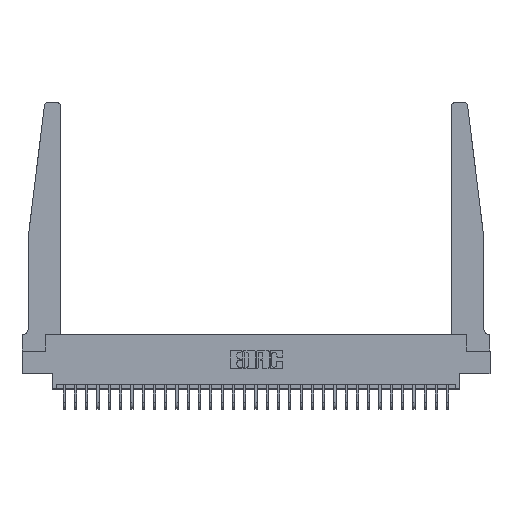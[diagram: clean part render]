
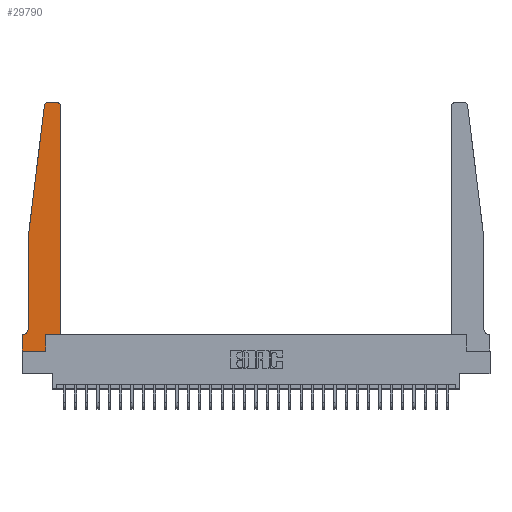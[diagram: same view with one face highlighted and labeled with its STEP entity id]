
A CAD part, top view. The second image highlights one B-rep face of the part: STEP entity #29790.
In plain terms, the highlighted planar face has unit normal (0, 0, 1).
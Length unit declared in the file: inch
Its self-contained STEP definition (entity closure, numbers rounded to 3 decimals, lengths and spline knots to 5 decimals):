
#77 = VERTEX_POINT ( 'NONE', #11737 ) ;
#547 = EDGE_CURVE ( 'NONE', #77, #27846, #12173, .T. ) ;
#548 = EDGE_CURVE ( 'NONE', #14902, #23360, #1290, .T. ) ;
#1290 = CIRCLE ( 'NONE', #2798, 0.05 ) ;
#1669 = VERTEX_POINT ( 'NONE', #28463 ) ;
#1721 = CARTESIAN_POINT ( 'NONE',  ( 0., 0., 0.37 ) ) ;
#1776 = VERTEX_POINT ( 'NONE', #9829 ) ;
#1814 = LINE ( 'NONE', #6059, #4827 ) ;
#1988 = CARTESIAN_POINT ( 'NONE',  ( 0.015, 0.1875, 0.37 ) ) ;
#2604 = CARTESIAN_POINT ( 'NONE',  ( 0.2605, 0.18, 0.37 ) ) ;
#2612 = DIRECTION ( 'NONE',  ( 1., 0., 0. ) ) ;
#2775 = DIRECTION ( 'NONE',  ( -1., 0., 0. ) ) ;
#2783 = CARTESIAN_POINT ( 'NONE',  ( 0.065, 1.25, 0.37 ) ) ;
#2798 = AXIS2_PLACEMENT_3D ( 'NONE', #9671, #7027, #2775 ) ;
#3379 = VECTOR ( 'NONE', #17967, 39.37008 ) ;
#3815 = DIRECTION ( 'NONE',  ( -0.122, -0.992, 0. ) ) ;
#3979 = DIRECTION ( 'NONE',  ( 0., 0., 1. ) ) ;
#4219 = VECTOR ( 'NONE', #24325, 39.37008 ) ;
#4601 = LINE ( 'NONE', #14142, #19421 ) ;
#4827 = VECTOR ( 'NONE', #27498, 39.37008 ) ;
#5202 = VERTEX_POINT ( 'NONE', #7641 ) ;
#5393 = ORIENTED_EDGE ( 'NONE', *, *, #21184, .T. ) ;
#5679 = LINE ( 'NONE', #10084, #4219 ) ;
#6037 = VERTEX_POINT ( 'NONE', #11784 ) ;
#6059 = CARTESIAN_POINT ( 'NONE',  ( 0.425, 0.18, 0.37 ) ) ;
#6143 = VERTEX_POINT ( 'NONE', #24298 ) ;
#6217 = ORIENTED_EDGE ( 'NONE', *, *, #13107, .T. ) ;
#7027 = DIRECTION ( 'NONE',  ( 0., 0., -1. ) ) ;
#7080 = ORIENTED_EDGE ( 'NONE', *, *, #548, .T. ) ;
#7641 = CARTESIAN_POINT ( 'NONE',  ( 0.425, 2.72, 0.37 ) ) ;
#8408 = ORIENTED_EDGE ( 'NONE', *, *, #11188, .T. ) ;
#8711 = DIRECTION ( 'NONE',  ( 1., 0., 0. ) ) ;
#8847 = DIRECTION ( 'NONE',  ( 1., 0., 0. ) ) ;
#9671 = CARTESIAN_POINT ( 'NONE',  ( 0.015, 0.2375, 0.37 ) ) ;
#9829 = CARTESIAN_POINT ( 'NONE',  ( 0.425, 0.18, 0.37 ) ) ;
#9842 = DIRECTION ( 'NONE',  ( 0., -1., 0. ) ) ;
#10084 = CARTESIAN_POINT ( 'NONE',  ( 0.2605, 0.18, 0.37 ) ) ;
#10304 = VECTOR ( 'NONE', #14522, 39.37008 ) ;
#10609 = EDGE_LOOP ( 'NONE', ( #6217, #8408, #15575, #14055, #7080, #5393, #14186, #26317, #18173, #21879, #25087, #14890 ) ) ;
#11073 = CARTESIAN_POINT ( 'NONE',  ( 0.065, 0.2375, 0.37 ) ) ;
#11188 = EDGE_CURVE ( 'NONE', #1669, #6037, #17817, .T. ) ;
#11536 = CARTESIAN_POINT ( 'NONE',  ( 0., 0., 0.37 ) ) ;
#11737 = CARTESIAN_POINT ( 'NONE',  ( 0., 0.1875, 0.37 ) ) ;
#11784 = CARTESIAN_POINT ( 'NONE',  ( 0.24675, 2.72367, 0.37 ) ) ;
#12173 = LINE ( 'NONE', #17027, #10304 ) ;
#12188 = CIRCLE ( 'NONE', #16159, 0.03 ) ;
#13059 = LINE ( 'NONE', #29648, #27290 ) ;
#13107 = EDGE_CURVE ( 'NONE', #25360, #1669, #4601, .T. ) ;
#13254 = LINE ( 'NONE', #13563, #20280 ) ;
#13405 = CARTESIAN_POINT ( 'NONE',  ( 0.27653, 2.72, 0.37 ) ) ;
#13563 = CARTESIAN_POINT ( 'NONE',  ( 0.065, 0.1875, 0.37 ) ) ;
#14055 = ORIENTED_EDGE ( 'NONE', *, *, #26693, .T. ) ;
#14142 = CARTESIAN_POINT ( 'NONE',  ( 0.25, 2.75, 0.37 ) ) ;
#14186 = ORIENTED_EDGE ( 'NONE', *, *, #547, .T. ) ;
#14474 = CARTESIAN_POINT ( 'NONE',  ( 0.395, 2.75, 0.37 ) ) ;
#14522 = DIRECTION ( 'NONE',  ( 0., -1., 0. ) ) ;
#14890 = ORIENTED_EDGE ( 'NONE', *, *, #23978, .T. ) ;
#14902 = VERTEX_POINT ( 'NONE', #11073 ) ;
#15575 = ORIENTED_EDGE ( 'NONE', *, *, #27249, .T. ) ;
#16159 = AXIS2_PLACEMENT_3D ( 'NONE', #20714, #3979, #8847 ) ;
#16348 = DIRECTION ( 'NONE',  ( 0., 1., 0. ) ) ;
#17027 = CARTESIAN_POINT ( 'NONE',  ( 0., 0., 0.37 ) ) ;
#17817 = CIRCLE ( 'NONE', #28816, 0.03 ) ;
#17967 = DIRECTION ( 'NONE',  ( 1., 0., 0. ) ) ;
#18018 = CARTESIAN_POINT ( 'NONE',  ( 0.065, 1.25, 0.37 ) ) ;
#18173 = ORIENTED_EDGE ( 'NONE', *, *, #24184, .T. ) ;
#18324 = VERTEX_POINT ( 'NONE', #2604 ) ;
#19016 = LINE ( 'NONE', #25911, #21248 ) ;
#19421 = VECTOR ( 'NONE', #23691, 39.37008 ) ;
#19514 = CARTESIAN_POINT ( 'NONE',  ( 0., 0.1875, 0.37 ) ) ;
#20280 = VECTOR ( 'NONE', #23442, 39.37008 ) ;
#20714 = CARTESIAN_POINT ( 'NONE',  ( 0.395, 2.72, 0.37 ) ) ;
#21184 = EDGE_CURVE ( 'NONE', #23360, #77, #13254, .T. ) ;
#21248 = VECTOR ( 'NONE', #16348, 39.37008 ) ;
#21879 = ORIENTED_EDGE ( 'NONE', *, *, #28241, .T. ) ;
#23360 = VERTEX_POINT ( 'NONE', #1988 ) ;
#23370 = EDGE_CURVE ( 'NONE', #27846, #6143, #27963, .T. ) ;
#23442 = DIRECTION ( 'NONE',  ( -1., 0., 0. ) ) ;
#23691 = DIRECTION ( 'NONE',  ( -1., 0., 0. ) ) ;
#23896 = AXIS2_PLACEMENT_3D ( 'NONE', #19514, #29519, #2612 ) ;
#23978 = EDGE_CURVE ( 'NONE', #5202, #25360, #12188, .T. ) ;
#24149 = EDGE_CURVE ( 'NONE', #1776, #5202, #19016, .T. ) ;
#24184 = EDGE_CURVE ( 'NONE', #6143, #18324, #5679, .T. ) ;
#24298 = CARTESIAN_POINT ( 'NONE',  ( 0.2605, 0., 0.37 ) ) ;
#24325 = DIRECTION ( 'NONE',  ( 0., 1., 0. ) ) ;
#24373 = PLANE ( 'NONE',  #23896 ) ;
#24398 = LINE ( 'NONE', #2783, #27323 ) ;
#25087 = ORIENTED_EDGE ( 'NONE', *, *, #24149, .T. ) ;
#25360 = VERTEX_POINT ( 'NONE', #14474 ) ;
#25871 = VERTEX_POINT ( 'NONE', #18018 ) ;
#25911 = CARTESIAN_POINT ( 'NONE',  ( 0.425, 0.18, 0.37 ) ) ;
#26317 = ORIENTED_EDGE ( 'NONE', *, *, #23370, .T. ) ;
#26693 = EDGE_CURVE ( 'NONE', #25871, #14902, #24398, .T. ) ;
#27015 = FACE_OUTER_BOUND ( 'NONE', #10609, .T. ) ;
#27249 = EDGE_CURVE ( 'NONE', #6037, #25871, #13059, .T. ) ;
#27290 = VECTOR ( 'NONE', #3815, 39.37008 ) ;
#27323 = VECTOR ( 'NONE', #9842, 39.37008 ) ;
#27498 = DIRECTION ( 'NONE',  ( 1., 0., 0. ) ) ;
#27785 = DIRECTION ( 'NONE',  ( 0., 0., 1. ) ) ;
#27846 = VERTEX_POINT ( 'NONE', #1721 ) ;
#27963 = LINE ( 'NONE', #11536, #3379 ) ;
#28241 = EDGE_CURVE ( 'NONE', #18324, #1776, #1814, .T. ) ;
#28463 = CARTESIAN_POINT ( 'NONE',  ( 0.27653, 2.75, 0.37 ) ) ;
#28816 = AXIS2_PLACEMENT_3D ( 'NONE', #13405, #27785, #8711 ) ;
#29519 = DIRECTION ( 'NONE',  ( 0., 0., 1. ) ) ;
#29648 = CARTESIAN_POINT ( 'NONE',  ( 0.065, 1.25, 0.37 ) ) ;
#29790 = ADVANCED_FACE ( 'NONE', ( #27015 ), #24373, .T. ) ;
